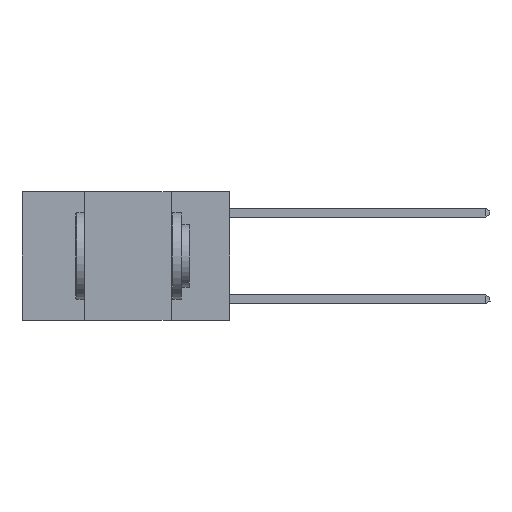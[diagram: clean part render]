
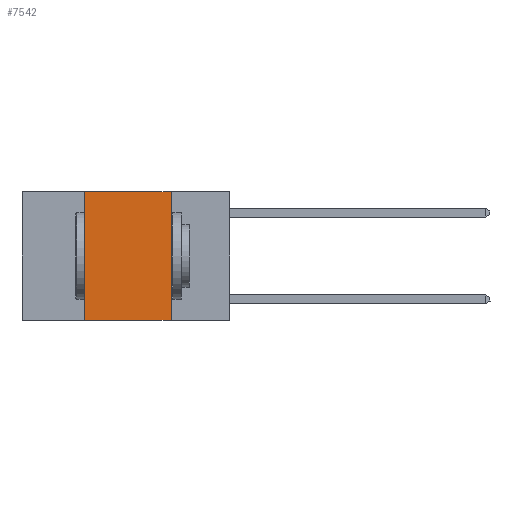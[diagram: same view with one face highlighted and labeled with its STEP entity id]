
A CAD part, left-side view. The second image highlights one B-rep face of the part: STEP entity #7542.
In plain terms, the highlighted planar face has unit normal (-1, 0, 0).
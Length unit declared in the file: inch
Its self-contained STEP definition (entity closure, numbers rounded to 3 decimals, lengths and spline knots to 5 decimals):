
#668 = DIRECTION ( 'NONE',  ( 0., 0., 1. ) ) ;
#1364 = VECTOR ( 'NONE', #668, 39.37008 ) ;
#1736 = DIRECTION ( 'NONE',  ( 0., -1., 0. ) ) ;
#2065 = CARTESIAN_POINT ( 'NONE',  ( 0., 0.42, 0. ) ) ;
#2231 = VERTEX_POINT ( 'NONE', #15806 ) ;
#2252 = LINE ( 'NONE', #2065, #1364 ) ;
#2988 = VECTOR ( 'NONE', #17150, 39.37008 ) ;
#3182 = LINE ( 'NONE', #7183, #13771 ) ;
#3249 = AXIS2_PLACEMENT_3D ( 'NONE', #3648, #5015, #14698 ) ;
#3648 = CARTESIAN_POINT ( 'NONE',  ( 0., 0.6, 0. ) ) ;
#4075 = ORIENTED_EDGE ( 'NONE', *, *, #4467, .F. ) ;
#4383 = VECTOR ( 'NONE', #10846, 39.37008 ) ;
#4467 = EDGE_CURVE ( 'NONE', #6541, #11912, #2252, .T. ) ;
#5015 = DIRECTION ( 'NONE',  ( 1., 0., 0. ) ) ;
#5060 = CARTESIAN_POINT ( 'NONE',  ( 0., 0.42, 0. ) ) ;
#6541 = VERTEX_POINT ( 'NONE', #12700 ) ;
#7183 = CARTESIAN_POINT ( 'NONE',  ( 0., 0.6, 0. ) ) ;
#7267 = ORIENTED_EDGE ( 'NONE', *, *, #8767, .F. ) ;
#7542 = ADVANCED_FACE ( 'NONE', ( #8589 ), #11939, .F. ) ;
#8056 = CARTESIAN_POINT ( 'NONE',  ( 0., 0.17, 0. ) ) ;
#8131 = EDGE_CURVE ( 'NONE', #6541, #2231, #17612, .T. ) ;
#8589 = FACE_OUTER_BOUND ( 'NONE', #10113, .T. ) ;
#8767 = EDGE_CURVE ( 'NONE', #11912, #14762, #3182, .T. ) ;
#10113 = EDGE_LOOP ( 'NONE', ( #16993, #7267, #4075, #10724 ) ) ;
#10724 = ORIENTED_EDGE ( 'NONE', *, *, #8131, .T. ) ;
#10846 = DIRECTION ( 'NONE',  ( 0., 0., -1. ) ) ;
#11912 = VERTEX_POINT ( 'NONE', #5060 ) ;
#11939 = PLANE ( 'NONE',  #3249 ) ;
#12175 = LINE ( 'NONE', #8056, #4383 ) ;
#12700 = CARTESIAN_POINT ( 'NONE',  ( 0., 0.42, -0.37 ) ) ;
#13771 = VECTOR ( 'NONE', #1736, 39.37008 ) ;
#14698 = DIRECTION ( 'NONE',  ( 0., 0., -1. ) ) ;
#14762 = VERTEX_POINT ( 'NONE', #15257 ) ;
#15257 = CARTESIAN_POINT ( 'NONE',  ( 0., 0.17, 0. ) ) ;
#15806 = CARTESIAN_POINT ( 'NONE',  ( 0., 0.17, -0.37 ) ) ;
#15815 = CARTESIAN_POINT ( 'NONE',  ( 0., 0.6, -0.37 ) ) ;
#15903 = EDGE_CURVE ( 'NONE', #14762, #2231, #12175, .T. ) ;
#16993 = ORIENTED_EDGE ( 'NONE', *, *, #15903, .F. ) ;
#17150 = DIRECTION ( 'NONE',  ( 0., -1., 0. ) ) ;
#17612 = LINE ( 'NONE', #15815, #2988 ) ;
